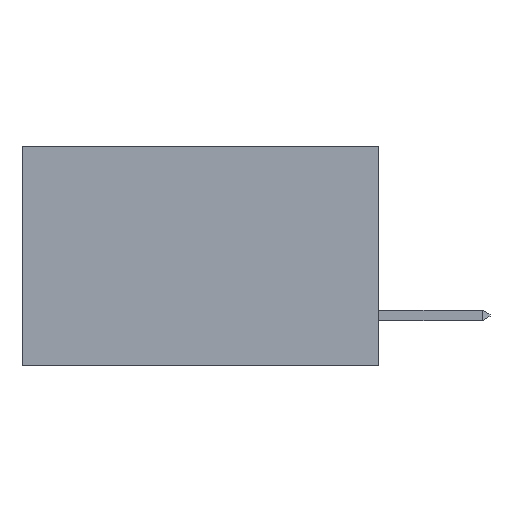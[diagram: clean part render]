
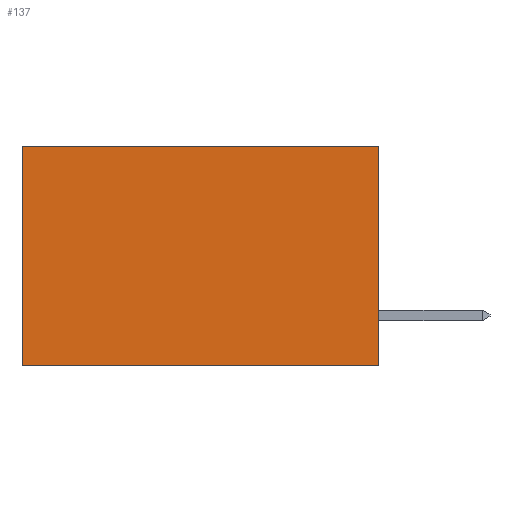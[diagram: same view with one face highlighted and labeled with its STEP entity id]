
A CAD part, left-side view. The second image highlights one B-rep face of the part: STEP entity #137.
In plain terms, the highlighted planar face has unit normal (-1, 0, 0).
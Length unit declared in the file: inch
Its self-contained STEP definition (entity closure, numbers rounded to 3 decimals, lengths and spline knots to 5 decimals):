
#126 = DIRECTION ( 'NONE',  ( 0., 1., 0. ) ) ;
#137 = ADVANCED_FACE ( 'NONE', ( #2256 ), #7618, .F. ) ;
#316 = CARTESIAN_POINT ( 'NONE',  ( 0.2615, 0., -0.37 ) ) ;
#842 = CARTESIAN_POINT ( 'NONE',  ( 0.2615, 0., 0. ) ) ;
#995 = LINE ( 'NONE', #316, #6605 ) ;
#1639 = VECTOR ( 'NONE', #2410, 39.37008 ) ;
#1791 = DIRECTION ( 'NONE',  ( 0., 0., -1. ) ) ;
#1856 = CARTESIAN_POINT ( 'NONE',  ( 0.2615, 0., -0.37 ) ) ;
#2026 = CARTESIAN_POINT ( 'NONE',  ( 0.2615, 0., 0. ) ) ;
#2256 = FACE_OUTER_BOUND ( 'NONE', #5583, .T. ) ;
#2410 = DIRECTION ( 'NONE',  ( 0., 1., 0. ) ) ;
#2512 = LINE ( 'NONE', #5825, #6144 ) ;
#2910 = VERTEX_POINT ( 'NONE', #842 ) ;
#4161 = EDGE_CURVE ( 'NONE', #8709, #5580, #995, .T. ) ;
#4617 = VERTEX_POINT ( 'NONE', #7563 ) ;
#4667 = EDGE_CURVE ( 'NONE', #4617, #5580, #2512, .T. ) ;
#5580 = VERTEX_POINT ( 'NONE', #6712 ) ;
#5583 = EDGE_LOOP ( 'NONE', ( #7504, #7599, #7704, #7916 ) ) ;
#5603 = DIRECTION ( 'NONE',  ( 0., 0., -1. ) ) ;
#5825 = CARTESIAN_POINT ( 'NONE',  ( 0.2615, 0.6, -0.37 ) ) ;
#6026 = EDGE_CURVE ( 'NONE', #2910, #8709, #8310, .T. ) ;
#6144 = VECTOR ( 'NONE', #5603, 39.37008 ) ;
#6605 = VECTOR ( 'NONE', #126, 39.37008 ) ;
#6626 = DIRECTION ( 'NONE',  ( 1., 0., 0. ) ) ;
#6712 = CARTESIAN_POINT ( 'NONE',  ( 0.2615, 0.6, -0.37 ) ) ;
#6779 = AXIS2_PLACEMENT_3D ( 'NONE', #7141, #6626, #7606 ) ;
#6805 = VECTOR ( 'NONE', #1791, 39.37008 ) ;
#6912 = CARTESIAN_POINT ( 'NONE',  ( 0.2615, 0., -0.37 ) ) ;
#7141 = CARTESIAN_POINT ( 'NONE',  ( 0.2615, 0., -0.37 ) ) ;
#7504 = ORIENTED_EDGE ( 'NONE', *, *, #4667, .T. ) ;
#7563 = CARTESIAN_POINT ( 'NONE',  ( 0.2615, 0.6, 0. ) ) ;
#7591 = LINE ( 'NONE', #2026, #1639 ) ;
#7599 = ORIENTED_EDGE ( 'NONE', *, *, #4161, .F. ) ;
#7606 = DIRECTION ( 'NONE',  ( 0., 0., -1. ) ) ;
#7618 = PLANE ( 'NONE',  #6779 ) ;
#7704 = ORIENTED_EDGE ( 'NONE', *, *, #6026, .F. ) ;
#7916 = ORIENTED_EDGE ( 'NONE', *, *, #8000, .T. ) ;
#8000 = EDGE_CURVE ( 'NONE', #2910, #4617, #7591, .T. ) ;
#8310 = LINE ( 'NONE', #1856, #6805 ) ;
#8709 = VERTEX_POINT ( 'NONE', #6912 ) ;
